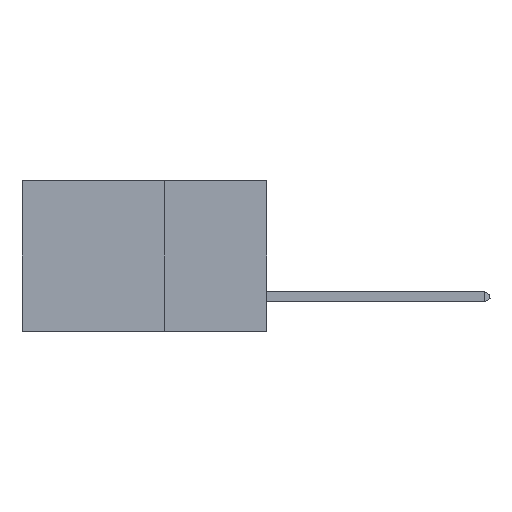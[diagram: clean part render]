
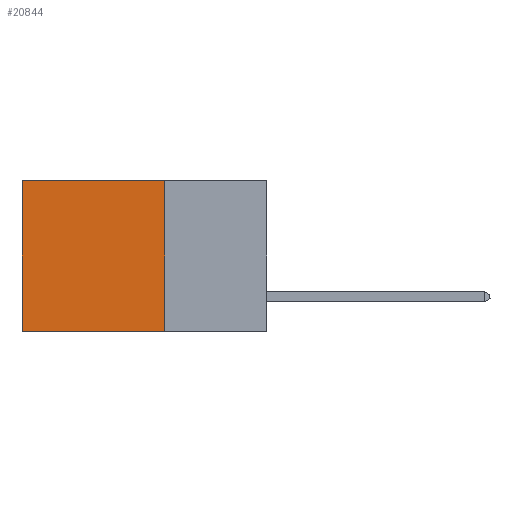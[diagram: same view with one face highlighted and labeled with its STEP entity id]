
A CAD part, left-side view. The second image highlights one B-rep face of the part: STEP entity #20844.
In plain terms, the highlighted planar face has unit normal (-1, 0, 0).
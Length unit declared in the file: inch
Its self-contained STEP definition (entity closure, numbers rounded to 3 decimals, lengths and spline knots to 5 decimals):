
#629 = VERTEX_POINT ( 'NONE', #4423 ) ;
#933 = DIRECTION ( 'NONE',  ( 0., 1., 0. ) ) ;
#2079 = CARTESIAN_POINT ( 'NONE',  ( 0.2875, 0.25, 0. ) ) ;
#2374 = LINE ( 'NONE', #16003, #22165 ) ;
#2514 = CARTESIAN_POINT ( 'NONE',  ( 0.2875, 0.25, -0.37 ) ) ;
#2876 = DIRECTION ( 'NONE',  ( 0., 0., -1. ) ) ;
#4423 = CARTESIAN_POINT ( 'NONE',  ( 0.2875, 0.25, -0.37 ) ) ;
#4983 = LINE ( 'NONE', #22681, #20303 ) ;
#6967 = EDGE_CURVE ( 'NONE', #8430, #11837, #2374, .T. ) ;
#7433 = DIRECTION ( 'NONE',  ( 0., 0., -1. ) ) ;
#7486 = VERTEX_POINT ( 'NONE', #20509 ) ;
#8430 = VERTEX_POINT ( 'NONE', #21814 ) ;
#8789 = VECTOR ( 'NONE', #933, 39.37008 ) ;
#9113 = ORIENTED_EDGE ( 'NONE', *, *, #6967, .T. ) ;
#9285 = LINE ( 'NONE', #2079, #13157 ) ;
#9769 = ORIENTED_EDGE ( 'NONE', *, *, #17401, .F. ) ;
#10534 = CARTESIAN_POINT ( 'NONE',  ( 0.2875, 0.25, 0. ) ) ;
#11837 = VERTEX_POINT ( 'NONE', #19479 ) ;
#12196 = DIRECTION ( 'NONE',  ( 1., 0., 0. ) ) ;
#13157 = VECTOR ( 'NONE', #15228, 39.37008 ) ;
#13238 = EDGE_CURVE ( 'NONE', #11837, #7486, #4983, .T. ) ;
#14302 = PLANE ( 'NONE',  #15465 ) ;
#15228 = DIRECTION ( 'NONE',  ( 0., 0., -1. ) ) ;
#15465 = AXIS2_PLACEMENT_3D ( 'NONE', #10534, #12196, #2876 ) ;
#16003 = CARTESIAN_POINT ( 'NONE',  ( 0.2875, 0.25, 0. ) ) ;
#16135 = EDGE_CURVE ( 'NONE', #629, #7486, #20760, .T. ) ;
#16483 = ORIENTED_EDGE ( 'NONE', *, *, #16135, .F. ) ;
#17401 = EDGE_CURVE ( 'NONE', #8430, #629, #9285, .T. ) ;
#18041 = DIRECTION ( 'NONE',  ( 0., 1., 0. ) ) ;
#19479 = CARTESIAN_POINT ( 'NONE',  ( 0.2875, 0.6, 0. ) ) ;
#19898 = EDGE_LOOP ( 'NONE', ( #23522, #16483, #9769, #9113 ) ) ;
#20303 = VECTOR ( 'NONE', #7433, 39.37008 ) ;
#20509 = CARTESIAN_POINT ( 'NONE',  ( 0.2875, 0.6, -0.37 ) ) ;
#20760 = LINE ( 'NONE', #2514, #8789 ) ;
#20844 = ADVANCED_FACE ( 'NONE', ( #23333 ), #14302, .F. ) ;
#21814 = CARTESIAN_POINT ( 'NONE',  ( 0.2875, 0.25, 0. ) ) ;
#22165 = VECTOR ( 'NONE', #18041, 39.37008 ) ;
#22681 = CARTESIAN_POINT ( 'NONE',  ( 0.2875, 0.6, 0. ) ) ;
#23333 = FACE_OUTER_BOUND ( 'NONE', #19898, .T. ) ;
#23522 = ORIENTED_EDGE ( 'NONE', *, *, #13238, .T. ) ;
